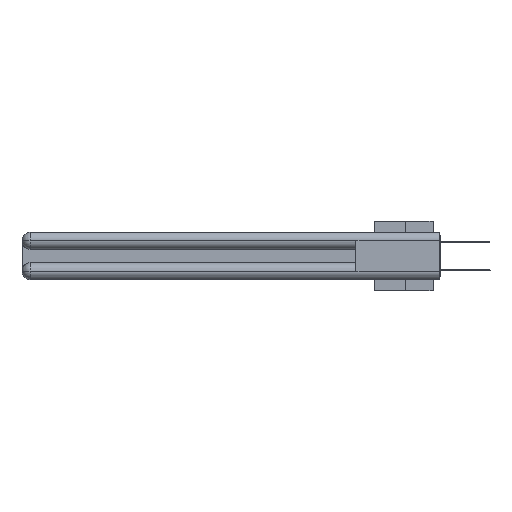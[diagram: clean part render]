
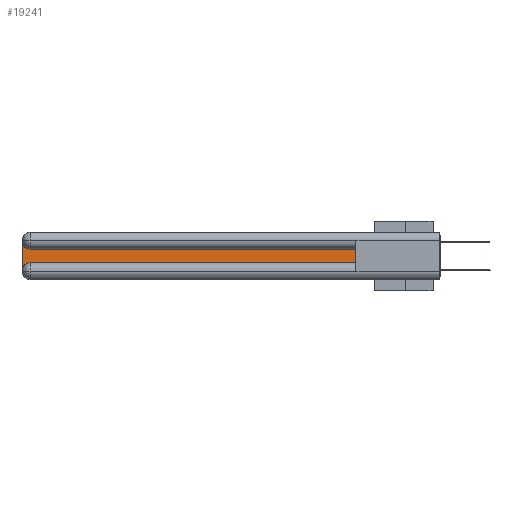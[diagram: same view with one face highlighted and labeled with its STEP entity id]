
A CAD part, left-side view. The second image highlights one B-rep face of the part: STEP entity #19241.
In plain terms, the highlighted planar face has unit normal (-1, 0, 0).
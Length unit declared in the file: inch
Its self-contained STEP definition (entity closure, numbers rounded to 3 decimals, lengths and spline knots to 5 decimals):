
#205 = VECTOR ( 'NONE', #12521, 39.37008 ) ;
#307 = VERTEX_POINT ( 'NONE', #14539 ) ;
#590 = CARTESIAN_POINT ( 'NONE',  ( 0.075, 0.6, -0.2175 ) ) ;
#707 = VERTEX_POINT ( 'NONE', #28166 ) ;
#1078 = ORIENTED_EDGE ( 'NONE', *, *, #30630, .T. ) ;
#2341 = EDGE_CURVE ( 'NONE', #19567, #8412, #13730, .T. ) ;
#3458 = EDGE_CURVE ( 'NONE', #12313, #307, #24359, .T. ) ;
#4566 = AXIS2_PLACEMENT_3D ( 'NONE', #10494, #29771, #17348 ) ;
#6249 = ORIENTED_EDGE ( 'NONE', *, *, #3458, .T. ) ;
#6432 = DIRECTION ( 'NONE',  ( 1., 0., 0. ) ) ;
#7124 = DIRECTION ( 'NONE',  ( 0., 1., 0. ) ) ;
#7922 = CARTESIAN_POINT ( 'NONE',  ( 0.075, 2.94, -0.1225 ) ) ;
#8412 = VERTEX_POINT ( 'NONE', #590 ) ;
#8538 = VERTEX_POINT ( 'NONE', #12865 ) ;
#8588 = LINE ( 'NONE', #24798, #205 ) ;
#9939 = VECTOR ( 'NONE', #30642, 39.37008 ) ;
#10494 = CARTESIAN_POINT ( 'NONE',  ( 0.075, 2.94, -0.0625 ) ) ;
#10521 = LINE ( 'NONE', #17489, #24665 ) ;
#11508 = EDGE_CURVE ( 'NONE', #8538, #12313, #18940, .T. ) ;
#11577 = DIRECTION ( 'NONE',  ( 1., 0., 0. ) ) ;
#11583 = FACE_OUTER_BOUND ( 'NONE', #12063, .T. ) ;
#11875 = CARTESIAN_POINT ( 'NONE',  ( 0.075, 0.6, -0.1225 ) ) ;
#12063 = EDGE_LOOP ( 'NONE', ( #31523, #6249, #14364, #1078, #30184, #22249 ) ) ;
#12313 = VERTEX_POINT ( 'NONE', #7922 ) ;
#12521 = DIRECTION ( 'NONE',  ( 0., 0., 1. ) ) ;
#12865 = CARTESIAN_POINT ( 'NONE',  ( 0.075, 0.6, -0.1225 ) ) ;
#12876 = EDGE_CURVE ( 'NONE', #8412, #8538, #8588, .T. ) ;
#12891 = AXIS2_PLACEMENT_3D ( 'NONE', #30899, #11577, #28651 ) ;
#13730 = LINE ( 'NONE', #18340, #9939 ) ;
#14035 = DIRECTION ( 'NONE',  ( 0., 0., -1. ) ) ;
#14364 = ORIENTED_EDGE ( 'NONE', *, *, #30403, .T. ) ;
#14539 = CARTESIAN_POINT ( 'NONE',  ( 0.075, 3., -0.0625 ) ) ;
#15414 = DIRECTION ( 'NONE',  ( 0., 0., -1. ) ) ;
#17348 = DIRECTION ( 'NONE',  ( 0., 0., -1. ) ) ;
#17484 = AXIS2_PLACEMENT_3D ( 'NONE', #18429, #6432, #14035 ) ;
#17489 = CARTESIAN_POINT ( 'NONE',  ( 0.075, 3., -0.2175 ) ) ;
#18340 = CARTESIAN_POINT ( 'NONE',  ( 0.075, 0.6, -0.2175 ) ) ;
#18429 = CARTESIAN_POINT ( 'NONE',  ( 0.075, 2.94, -0.2775 ) ) ;
#18862 = CARTESIAN_POINT ( 'NONE',  ( 0.075, 2.94, -0.2175 ) ) ;
#18940 = LINE ( 'NONE', #11875, #24673 ) ;
#19241 = ADVANCED_FACE ( 'NONE', ( #11583 ), #31106, .F. ) ;
#19567 = VERTEX_POINT ( 'NONE', #18862 ) ;
#22249 = ORIENTED_EDGE ( 'NONE', *, *, #12876, .T. ) ;
#24359 = CIRCLE ( 'NONE', #4566, 0.06 ) ;
#24665 = VECTOR ( 'NONE', #15414, 39.37008 ) ;
#24673 = VECTOR ( 'NONE', #7124, 39.37008 ) ;
#24798 = CARTESIAN_POINT ( 'NONE',  ( 0.075, 0.6, -0.2175 ) ) ;
#28166 = CARTESIAN_POINT ( 'NONE',  ( 0.075, 3., -0.2775 ) ) ;
#28651 = DIRECTION ( 'NONE',  ( 0., 0., -1. ) ) ;
#29771 = DIRECTION ( 'NONE',  ( 1., 0., 0. ) ) ;
#30044 = CIRCLE ( 'NONE', #17484, 0.06 ) ;
#30184 = ORIENTED_EDGE ( 'NONE', *, *, #2341, .T. ) ;
#30403 = EDGE_CURVE ( 'NONE', #307, #707, #10521, .T. ) ;
#30630 = EDGE_CURVE ( 'NONE', #707, #19567, #30044, .T. ) ;
#30642 = DIRECTION ( 'NONE',  ( 0., -1., 0. ) ) ;
#30899 = CARTESIAN_POINT ( 'NONE',  ( 0.075, 3., -0.1225 ) ) ;
#31106 = PLANE ( 'NONE',  #12891 ) ;
#31523 = ORIENTED_EDGE ( 'NONE', *, *, #11508, .T. ) ;
